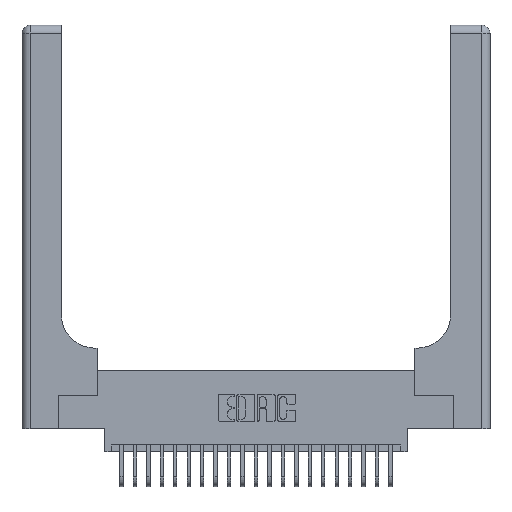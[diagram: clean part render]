
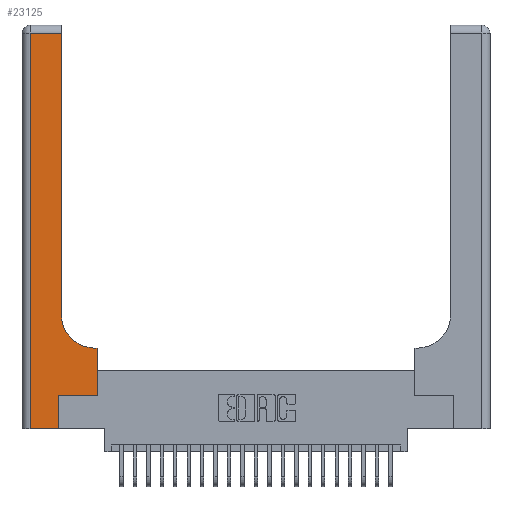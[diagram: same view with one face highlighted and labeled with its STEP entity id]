
A CAD part, top view. The second image highlights one B-rep face of the part: STEP entity #23125.
In plain terms, the highlighted planar face has unit normal (0, 0, 1).
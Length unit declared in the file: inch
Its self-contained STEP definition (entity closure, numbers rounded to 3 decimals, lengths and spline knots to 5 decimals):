
#486 = LINE ( 'NONE', #9259, #13185 ) ;
#1773 = LINE ( 'NONE', #21229, #13857 ) ;
#2097 = ORIENTED_EDGE ( 'NONE', *, *, #8297, .T. ) ;
#2121 = CARTESIAN_POINT ( 'NONE',  ( 0.2915, 2.94, 0.37 ) ) ;
#2657 = DIRECTION ( 'NONE',  ( 1., 0., 0. ) ) ;
#2722 = VERTEX_POINT ( 'NONE', #2818 ) ;
#2818 = CARTESIAN_POINT ( 'NONE',  ( 0.5585, 0.6, 0.37 ) ) ;
#3285 = DIRECTION ( 'NONE',  ( 1., 0., 0. ) ) ;
#3778 = ORIENTED_EDGE ( 'NONE', *, *, #12074, .T. ) ;
#3988 = DIRECTION ( 'NONE',  ( -1., 0., 0. ) ) ;
#4057 = EDGE_CURVE ( 'NONE', #8906, #14710, #18904, .T. ) ;
#4203 = ORIENTED_EDGE ( 'NONE', *, *, #23967, .T. ) ;
#4767 = EDGE_CURVE ( 'NONE', #5611, #6267, #23980, .T. ) ;
#4999 = EDGE_LOOP ( 'NONE', ( #2097, #7856, #17970, #11721, #3778, #12049, #4203, #8877, #22466 ) ) ;
#5113 = AXIS2_PLACEMENT_3D ( 'NONE', #6003, #16268, #3988 ) ;
#5611 = VERTEX_POINT ( 'NONE', #22633 ) ;
#6003 = CARTESIAN_POINT ( 'NONE',  ( 0., 3., 0.37 ) ) ;
#6267 = VERTEX_POINT ( 'NONE', #11194 ) ;
#6844 = CARTESIAN_POINT ( 'NONE',  ( 0.2915, 3., 0.37 ) ) ;
#7856 = ORIENTED_EDGE ( 'NONE', *, *, #26184, .T. ) ;
#8004 = VERTEX_POINT ( 'NONE', #24637 ) ;
#8297 = EDGE_CURVE ( 'NONE', #6267, #26064, #18117, .T. ) ;
#8690 = CARTESIAN_POINT ( 'NONE',  ( 0.269, 0.25, 0.37 ) ) ;
#8860 = CARTESIAN_POINT ( 'NONE',  ( 0., 2.94, 0.37 ) ) ;
#8877 = ORIENTED_EDGE ( 'NONE', *, *, #18814, .T. ) ;
#8906 = VERTEX_POINT ( 'NONE', #13762 ) ;
#9259 = CARTESIAN_POINT ( 'NONE',  ( 0.269, 0., 0.37 ) ) ;
#9365 = EDGE_CURVE ( 'NONE', #10578, #8004, #23497, .T. ) ;
#9500 = EDGE_CURVE ( 'NONE', #21814, #8906, #20950, .T. ) ;
#9767 = DIRECTION ( 'NONE',  ( 1., 0., 0. ) ) ;
#10578 = VERTEX_POINT ( 'NONE', #17298 ) ;
#11194 = CARTESIAN_POINT ( 'NONE',  ( 0.2915, 0.85, 0.37 ) ) ;
#11336 = CARTESIAN_POINT ( 'NONE',  ( 0.06, 2.94, 0.37 ) ) ;
#11525 = FACE_OUTER_BOUND ( 'NONE', #4999, .T. ) ;
#11721 = ORIENTED_EDGE ( 'NONE', *, *, #4057, .T. ) ;
#12049 = ORIENTED_EDGE ( 'NONE', *, *, #9365, .T. ) ;
#12074 = EDGE_CURVE ( 'NONE', #14710, #10578, #486, .T. ) ;
#12526 = PLANE ( 'NONE',  #5113 ) ;
#13185 = VECTOR ( 'NONE', #13436, 39.37008 ) ;
#13436 = DIRECTION ( 'NONE',  ( 0., 1., 0. ) ) ;
#13530 = VECTOR ( 'NONE', #9767, 39.37008 ) ;
#13762 = CARTESIAN_POINT ( 'NONE',  ( 0.06, 0., 0.37 ) ) ;
#13857 = VECTOR ( 'NONE', #21847, 39.37008 ) ;
#14710 = VERTEX_POINT ( 'NONE', #15802 ) ;
#14911 = DIRECTION ( 'NONE',  ( -1., 0., 0. ) ) ;
#14986 = DIRECTION ( 'NONE',  ( 0., 1., 0. ) ) ;
#15371 = CARTESIAN_POINT ( 'NONE',  ( 0.06, 3., 0.37 ) ) ;
#15400 = CARTESIAN_POINT ( 'NONE',  ( 0.5415, 0.85, 0.37 ) ) ;
#15802 = CARTESIAN_POINT ( 'NONE',  ( 0.269, 0., 0.37 ) ) ;
#15908 = VECTOR ( 'NONE', #2657, 39.37008 ) ;
#16268 = DIRECTION ( 'NONE',  ( 0., 0., -1. ) ) ;
#16631 = DIRECTION ( 'NONE',  ( 0., 1., 0. ) ) ;
#17298 = CARTESIAN_POINT ( 'NONE',  ( 0.269, 0.25, 0.37 ) ) ;
#17970 = ORIENTED_EDGE ( 'NONE', *, *, #9500, .T. ) ;
#18009 = CARTESIAN_POINT ( 'NONE',  ( 0., 0., 0.37 ) ) ;
#18117 = LINE ( 'NONE', #6844, #23885 ) ;
#18463 = VECTOR ( 'NONE', #14986, 39.37008 ) ;
#18780 = LINE ( 'NONE', #20838, #18463 ) ;
#18814 = EDGE_CURVE ( 'NONE', #2722, #5611, #1773, .T. ) ;
#18904 = LINE ( 'NONE', #18009, #13530 ) ;
#19506 = DIRECTION ( 'NONE',  ( 0., -1., 0. ) ) ;
#19957 = VECTOR ( 'NONE', #14911, 39.37008 ) ;
#20272 = LINE ( 'NONE', #8860, #19957 ) ;
#20838 = CARTESIAN_POINT ( 'NONE',  ( 0.5585, 0.25, 0.37 ) ) ;
#20950 = LINE ( 'NONE', #15371, #24770 ) ;
#21229 = CARTESIAN_POINT ( 'NONE',  ( 0.2915, 0.6, 0.37 ) ) ;
#21814 = VERTEX_POINT ( 'NONE', #11336 ) ;
#21847 = DIRECTION ( 'NONE',  ( -1., 0., 0. ) ) ;
#22466 = ORIENTED_EDGE ( 'NONE', *, *, #4767, .T. ) ;
#22633 = CARTESIAN_POINT ( 'NONE',  ( 0.5415, 0.6, 0.37 ) ) ;
#23125 = ADVANCED_FACE ( 'NONE', ( #11525 ), #12526, .F. ) ;
#23497 = LINE ( 'NONE', #8690, #15908 ) ;
#23885 = VECTOR ( 'NONE', #16631, 39.37008 ) ;
#23895 = DIRECTION ( 'NONE',  ( 0., 0., -1. ) ) ;
#23967 = EDGE_CURVE ( 'NONE', #8004, #2722, #18780, .T. ) ;
#23980 = CIRCLE ( 'NONE', #25073, 0.25 ) ;
#24637 = CARTESIAN_POINT ( 'NONE',  ( 0.5585, 0.25, 0.37 ) ) ;
#24770 = VECTOR ( 'NONE', #19506, 39.37008 ) ;
#25073 = AXIS2_PLACEMENT_3D ( 'NONE', #15400, #23895, #3285 ) ;
#26064 = VERTEX_POINT ( 'NONE', #2121 ) ;
#26184 = EDGE_CURVE ( 'NONE', #26064, #21814, #20272, .T. ) ;
